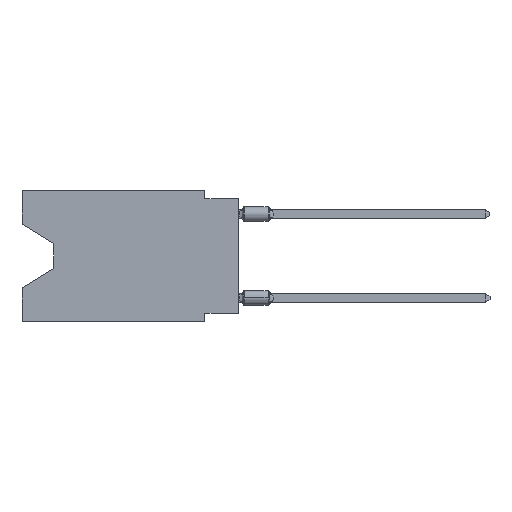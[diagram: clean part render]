
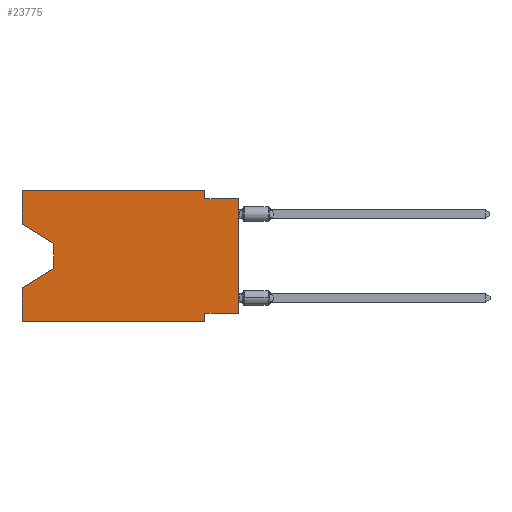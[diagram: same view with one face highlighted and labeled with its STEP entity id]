
A CAD part, left-side view. The second image highlights one B-rep face of the part: STEP entity #23775.
In plain terms, the highlighted planar face has unit normal (-1, 0, 0).
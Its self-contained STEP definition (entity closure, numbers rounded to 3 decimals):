
#333 = LINE ( 'NONE', #10869, #22887 ) ;
#668 = VERTEX_POINT ( 'NONE', #22591 ) ;
#723 = VERTEX_POINT ( 'NONE', #3602 ) ;
#1055 = DIRECTION ( 'NONE',  ( 0., 0., 1. ) ) ;
#2179 = CARTESIAN_POINT ( 'NONE',  ( 0., 16.383, -2.546 ) ) ;
#2746 = VECTOR ( 'NONE', #21847, 1000. ) ;
#3025 = VECTOR ( 'NONE', #20131, 1000. ) ;
#3089 = EDGE_CURVE ( 'NONE', #26769, #10326, #333, .T. ) ;
#3335 = ORIENTED_EDGE ( 'NONE', *, *, #3089, .F. ) ;
#3373 = LINE ( 'NONE', #21186, #12653 ) ;
#3598 = LINE ( 'NONE', #3759, #15990 ) ;
#3602 = CARTESIAN_POINT ( 'NONE',  ( 0., 16.383, -2.546 ) ) ;
#3646 = CARTESIAN_POINT ( 'NONE',  ( 0., 16.383, -9.906 ) ) ;
#3684 = ORIENTED_EDGE ( 'NONE', *, *, #18345, .F. ) ;
#3687 = ORIENTED_EDGE ( 'NONE', *, *, #22008, .T. ) ;
#3759 = CARTESIAN_POINT ( 'NONE',  ( 0., 0., -9.271 ) ) ;
#4002 = ORIENTED_EDGE ( 'NONE', *, *, #29358, .F. ) ;
#4624 = CARTESIAN_POINT ( 'NONE',  ( 0., 2.54, 0. ) ) ;
#5418 = DIRECTION ( 'NONE',  ( 0., -1., 0. ) ) ;
#5548 = CARTESIAN_POINT ( 'NONE',  ( 0., 16.383, -7.36 ) ) ;
#5743 = LINE ( 'NONE', #26037, #23892 ) ;
#5908 = LINE ( 'NONE', #28345, #17320 ) ;
#6113 = CARTESIAN_POINT ( 'NONE',  ( 0., 13.97, -4.013 ) ) ;
#6823 = ORIENTED_EDGE ( 'NONE', *, *, #24522, .F. ) ;
#8848 = EDGE_CURVE ( 'NONE', #668, #27742, #31176, .T. ) ;
#9540 = DIRECTION ( 'NONE',  ( 1., 0., 0. ) ) ;
#9775 = CARTESIAN_POINT ( 'NONE',  ( 0., 16.383, -9.906 ) ) ;
#9846 = EDGE_LOOP ( 'NONE', ( #15984, #30263, #18709, #4002, #3687, #6823, #3684, #21877, #23815, #30139, #3335, #18366 ) ) ;
#10326 = VERTEX_POINT ( 'NONE', #4624 ) ;
#10869 = CARTESIAN_POINT ( 'NONE',  ( 0., 16.383, 0. ) ) ;
#11585 = VERTEX_POINT ( 'NONE', #22500 ) ;
#11618 = EDGE_CURVE ( 'NONE', #10326, #29079, #16881, .T. ) ;
#11732 = VERTEX_POINT ( 'NONE', #12582 ) ;
#12009 = CARTESIAN_POINT ( 'NONE',  ( 0., 16.383, 0. ) ) ;
#12234 = DIRECTION ( 'NONE',  ( 0., -0.855, -0.519 ) ) ;
#12438 = CARTESIAN_POINT ( 'NONE',  ( 0., 13.97, -5.893 ) ) ;
#12582 = CARTESIAN_POINT ( 'NONE',  ( 0., 2.54, -9.271 ) ) ;
#12653 = VECTOR ( 'NONE', #1055, 1000. ) ;
#12675 = LINE ( 'NONE', #28184, #23905 ) ;
#13161 = CARTESIAN_POINT ( 'NONE',  ( 0., 0., -0.635 ) ) ;
#13688 = DIRECTION ( 'NONE',  ( 0., -1., 0. ) ) ;
#14440 = VECTOR ( 'NONE', #17394, 1000. ) ;
#15012 = LINE ( 'NONE', #30669, #3025 ) ;
#15661 = DIRECTION ( 'NONE',  ( 0., -1., 0. ) ) ;
#15803 = DIRECTION ( 'NONE',  ( 0., 0., 1. ) ) ;
#15841 = DIRECTION ( 'NONE',  ( 0., 0., -1. ) ) ;
#15984 = ORIENTED_EDGE ( 'NONE', *, *, #28676, .T. ) ;
#15990 = VECTOR ( 'NONE', #21081, 1000. ) ;
#16175 = LINE ( 'NONE', #3646, #32516 ) ;
#16881 = LINE ( 'NONE', #24298, #2746 ) ;
#17320 = VECTOR ( 'NONE', #23391, 1000. ) ;
#17394 = DIRECTION ( 'NONE',  ( 0., 0.855, -0.519 ) ) ;
#17870 = LINE ( 'NONE', #12438, #14440 ) ;
#18169 = EDGE_CURVE ( 'NONE', #29079, #18219, #12675, .T. ) ;
#18219 = VERTEX_POINT ( 'NONE', #13161 ) ;
#18345 = EDGE_CURVE ( 'NONE', #11585, #11732, #3598, .T. ) ;
#18366 = ORIENTED_EDGE ( 'NONE', *, *, #23417, .F. ) ;
#18667 = VERTEX_POINT ( 'NONE', #5548 ) ;
#18709 = ORIENTED_EDGE ( 'NONE', *, *, #19073, .T. ) ;
#18736 = VERTEX_POINT ( 'NONE', #30124 ) ;
#18967 = CARTESIAN_POINT ( 'NONE',  ( 0., 2.54, -0.635 ) ) ;
#19073 = EDGE_CURVE ( 'NONE', #27742, #18667, #17870, .T. ) ;
#19843 = LINE ( 'NONE', #2179, #30725 ) ;
#19913 = AXIS2_PLACEMENT_3D ( 'NONE', #12009, #9540, #22247 ) ;
#20131 = DIRECTION ( 'NONE',  ( 0., 0., 1. ) ) ;
#21081 = DIRECTION ( 'NONE',  ( 0., 1., 0. ) ) ;
#21186 = CARTESIAN_POINT ( 'NONE',  ( 0., 0., 0. ) ) ;
#21686 = CARTESIAN_POINT ( 'NONE',  ( 0., 13.97, -5.893 ) ) ;
#21706 = VERTEX_POINT ( 'NONE', #9775 ) ;
#21847 = DIRECTION ( 'NONE',  ( 0., 0., -1. ) ) ;
#21877 = ORIENTED_EDGE ( 'NONE', *, *, #26474, .T. ) ;
#22008 = EDGE_CURVE ( 'NONE', #21706, #18736, #16175, .T. ) ;
#22247 = DIRECTION ( 'NONE',  ( 0., 0., -1. ) ) ;
#22500 = CARTESIAN_POINT ( 'NONE',  ( 0., 0., -9.271 ) ) ;
#22591 = CARTESIAN_POINT ( 'NONE',  ( 0., 13.97, -4.013 ) ) ;
#22887 = VECTOR ( 'NONE', #15661, 1000. ) ;
#23391 = DIRECTION ( 'NONE',  ( 0., 0., -1. ) ) ;
#23417 = EDGE_CURVE ( 'NONE', #723, #26769, #15012, .T. ) ;
#23663 = VECTOR ( 'NONE', #15841, 1000. ) ;
#23775 = ADVANCED_FACE ( 'NONE', ( #29171 ), #32296, .F. ) ;
#23815 = ORIENTED_EDGE ( 'NONE', *, *, #18169, .F. ) ;
#23892 = VECTOR ( 'NONE', #15803, 1000. ) ;
#23905 = VECTOR ( 'NONE', #5418, 1000. ) ;
#24298 = CARTESIAN_POINT ( 'NONE',  ( 0., 2.54, 0. ) ) ;
#24522 = EDGE_CURVE ( 'NONE', #11732, #18736, #5908, .T. ) ;
#26037 = CARTESIAN_POINT ( 'NONE',  ( 0., 16.383, 0. ) ) ;
#26474 = EDGE_CURVE ( 'NONE', #11585, #18219, #3373, .T. ) ;
#26769 = VERTEX_POINT ( 'NONE', #30389 ) ;
#27742 = VERTEX_POINT ( 'NONE', #21686 ) ;
#28184 = CARTESIAN_POINT ( 'NONE',  ( 0., 0., -0.635 ) ) ;
#28345 = CARTESIAN_POINT ( 'NONE',  ( 0., 2.54, -9.906 ) ) ;
#28676 = EDGE_CURVE ( 'NONE', #723, #668, #19843, .T. ) ;
#29079 = VERTEX_POINT ( 'NONE', #18967 ) ;
#29171 = FACE_OUTER_BOUND ( 'NONE', #9846, .T. ) ;
#29358 = EDGE_CURVE ( 'NONE', #21706, #18667, #5743, .T. ) ;
#30124 = CARTESIAN_POINT ( 'NONE',  ( 0., 2.54, -9.906 ) ) ;
#30139 = ORIENTED_EDGE ( 'NONE', *, *, #11618, .F. ) ;
#30263 = ORIENTED_EDGE ( 'NONE', *, *, #8848, .T. ) ;
#30389 = CARTESIAN_POINT ( 'NONE',  ( 0., 16.383, 0. ) ) ;
#30669 = CARTESIAN_POINT ( 'NONE',  ( 0., 16.383, 0. ) ) ;
#30725 = VECTOR ( 'NONE', #12234, 1000. ) ;
#31176 = LINE ( 'NONE', #6113, #23663 ) ;
#32296 = PLANE ( 'NONE',  #19913 ) ;
#32516 = VECTOR ( 'NONE', #13688, 1000. ) ;
